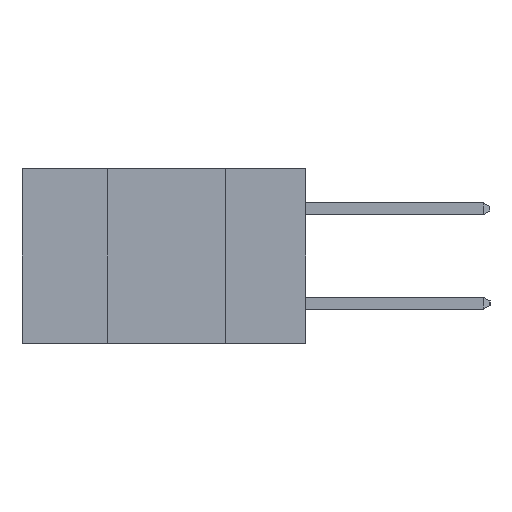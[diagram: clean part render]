
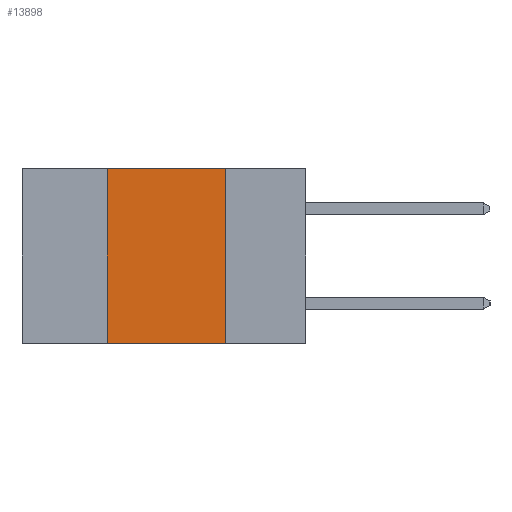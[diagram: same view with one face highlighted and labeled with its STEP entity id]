
A CAD part, left-side view. The second image highlights one B-rep face of the part: STEP entity #13898.
In plain terms, the highlighted planar face has unit normal (-1, 0, 0).
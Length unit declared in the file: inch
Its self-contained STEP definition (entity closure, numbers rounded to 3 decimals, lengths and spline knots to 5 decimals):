
#609 = CARTESIAN_POINT ( 'NONE',  ( 0., 0.17, -0.37 ) ) ;
#2079 = CARTESIAN_POINT ( 'NONE',  ( 0., 0.6, 0. ) ) ;
#2204 = EDGE_LOOP ( 'NONE', ( #14368, #11187, #12289, #4789 ) ) ;
#3043 = DIRECTION ( 'NONE',  ( 1., 0., 0. ) ) ;
#3296 = VECTOR ( 'NONE', #8826, 39.37008 ) ;
#3450 = VERTEX_POINT ( 'NONE', #609 ) ;
#3685 = DIRECTION ( 'NONE',  ( 0., -1., 0. ) ) ;
#3713 = VECTOR ( 'NONE', #17492, 39.37008 ) ;
#3793 = VECTOR ( 'NONE', #4404, 39.37008 ) ;
#3862 = VECTOR ( 'NONE', #3685, 39.37008 ) ;
#4337 = CARTESIAN_POINT ( 'NONE',  ( 0., 0.17, -0.37 ) ) ;
#4364 = LINE ( 'NONE', #2079, #3862 ) ;
#4404 = DIRECTION ( 'NONE',  ( 0., 0., -1. ) ) ;
#4428 = VERTEX_POINT ( 'NONE', #20380 ) ;
#4789 = ORIENTED_EDGE ( 'NONE', *, *, #11692, .T. ) ;
#6443 = VERTEX_POINT ( 'NONE', #11998 ) ;
#8758 = CARTESIAN_POINT ( 'NONE',  ( 0., 0.42, -0.37 ) ) ;
#8826 = DIRECTION ( 'NONE',  ( 0., 0., 1. ) ) ;
#8883 = FACE_OUTER_BOUND ( 'NONE', #2204, .T. ) ;
#9534 = EDGE_CURVE ( 'NONE', #10476, #4428, #19668, .T. ) ;
#9942 = EDGE_CURVE ( 'NONE', #6443, #3450, #16465, .T. ) ;
#10027 = CARTESIAN_POINT ( 'NONE',  ( 0., 0.42, -0.37 ) ) ;
#10385 = AXIS2_PLACEMENT_3D ( 'NONE', #17293, #3043, #14206 ) ;
#10476 = VERTEX_POINT ( 'NONE', #10027 ) ;
#11187 = ORIENTED_EDGE ( 'NONE', *, *, #14168, .F. ) ;
#11692 = EDGE_CURVE ( 'NONE', #10476, #3450, #13215, .T. ) ;
#11998 = CARTESIAN_POINT ( 'NONE',  ( 0., 0.17, 0. ) ) ;
#12289 = ORIENTED_EDGE ( 'NONE', *, *, #9534, .F. ) ;
#12648 = PLANE ( 'NONE',  #10385 ) ;
#13215 = LINE ( 'NONE', #17458, #3713 ) ;
#13898 = ADVANCED_FACE ( 'NONE', ( #8883 ), #12648, .F. ) ;
#14168 = EDGE_CURVE ( 'NONE', #4428, #6443, #4364, .T. ) ;
#14206 = DIRECTION ( 'NONE',  ( 0., 0., -1. ) ) ;
#14368 = ORIENTED_EDGE ( 'NONE', *, *, #9942, .F. ) ;
#16465 = LINE ( 'NONE', #4337, #3793 ) ;
#17293 = CARTESIAN_POINT ( 'NONE',  ( 0., 0.6, 0. ) ) ;
#17458 = CARTESIAN_POINT ( 'NONE',  ( 0., 0.6, -0.37 ) ) ;
#17492 = DIRECTION ( 'NONE',  ( 0., -1., 0. ) ) ;
#19668 = LINE ( 'NONE', #8758, #3296 ) ;
#20380 = CARTESIAN_POINT ( 'NONE',  ( 0., 0.42, 0. ) ) ;
